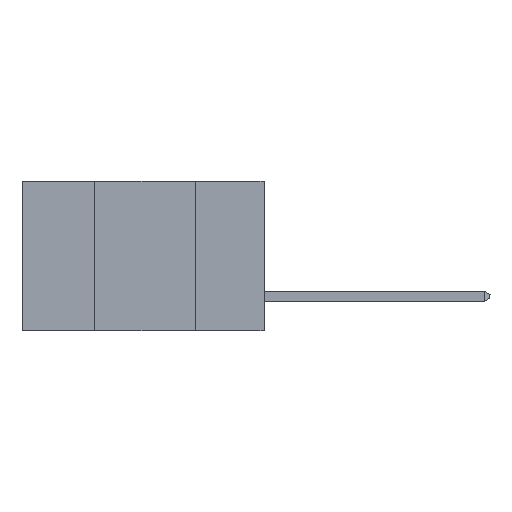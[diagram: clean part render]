
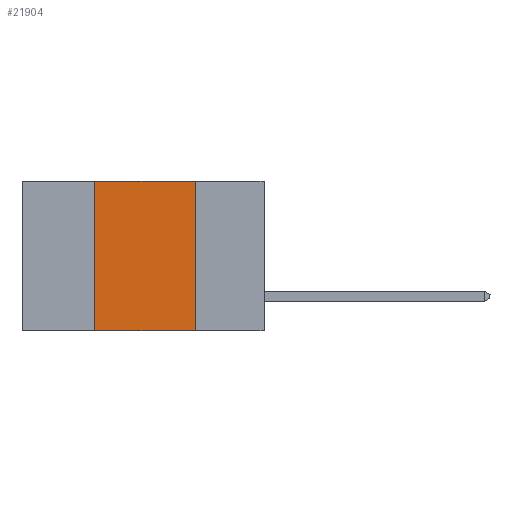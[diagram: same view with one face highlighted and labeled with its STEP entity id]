
A CAD part, left-side view. The second image highlights one B-rep face of the part: STEP entity #21904.
In plain terms, the highlighted planar face has unit normal (-1, 0, 0).
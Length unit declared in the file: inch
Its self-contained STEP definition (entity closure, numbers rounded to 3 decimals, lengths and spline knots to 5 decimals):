
#374 = VERTEX_POINT ( 'NONE', #4082 ) ;
#477 = DIRECTION ( 'NONE',  ( 0., -1., 0. ) ) ;
#605 = DIRECTION ( 'NONE',  ( 0., 0., -1. ) ) ;
#688 = EDGE_CURVE ( 'NONE', #2440, #374, #1144, .T. ) ;
#1144 = LINE ( 'NONE', #6631, #23413 ) ;
#1272 = ORIENTED_EDGE ( 'NONE', *, *, #688, .T. ) ;
#1585 = VECTOR ( 'NONE', #17593, 39.37008 ) ;
#1866 = EDGE_CURVE ( 'NONE', #2440, #13167, #24547, .T. ) ;
#2440 = VERTEX_POINT ( 'NONE', #23656 ) ;
#2526 = CARTESIAN_POINT ( 'NONE',  ( 0., 0.42, 0. ) ) ;
#2597 = LINE ( 'NONE', #20022, #15377 ) ;
#2714 = EDGE_LOOP ( 'NONE', ( #3973, #21644, #3188, #1272 ) ) ;
#3188 = ORIENTED_EDGE ( 'NONE', *, *, #1866, .F. ) ;
#3973 = ORIENTED_EDGE ( 'NONE', *, *, #20418, .F. ) ;
#4069 = VERTEX_POINT ( 'NONE', #12179 ) ;
#4082 = CARTESIAN_POINT ( 'NONE',  ( 0., 0.17, -0.37 ) ) ;
#4634 = CARTESIAN_POINT ( 'NONE',  ( 0., 0.6, 0. ) ) ;
#5079 = FACE_OUTER_BOUND ( 'NONE', #2714, .T. ) ;
#5147 = EDGE_CURVE ( 'NONE', #13167, #4069, #2597, .T. ) ;
#6631 = CARTESIAN_POINT ( 'NONE',  ( 0., 0.6, -0.37 ) ) ;
#7844 = LINE ( 'NONE', #13879, #1585 ) ;
#8522 = CARTESIAN_POINT ( 'NONE',  ( 0., 0.42, 0. ) ) ;
#8560 = AXIS2_PLACEMENT_3D ( 'NONE', #4634, #23311, #605 ) ;
#10403 = DIRECTION ( 'NONE',  ( 0., 0., 1. ) ) ;
#12096 = PLANE ( 'NONE',  #8560 ) ;
#12179 = CARTESIAN_POINT ( 'NONE',  ( 0., 0.17, 0. ) ) ;
#13167 = VERTEX_POINT ( 'NONE', #8522 ) ;
#13879 = CARTESIAN_POINT ( 'NONE',  ( 0., 0.17, 0. ) ) ;
#15377 = VECTOR ( 'NONE', #477, 39.37008 ) ;
#17403 = VECTOR ( 'NONE', #10403, 39.37008 ) ;
#17593 = DIRECTION ( 'NONE',  ( 0., 0., -1. ) ) ;
#20022 = CARTESIAN_POINT ( 'NONE',  ( 0., 0.6, 0. ) ) ;
#20418 = EDGE_CURVE ( 'NONE', #4069, #374, #7844, .T. ) ;
#21644 = ORIENTED_EDGE ( 'NONE', *, *, #5147, .F. ) ;
#21904 = ADVANCED_FACE ( 'NONE', ( #5079 ), #12096, .F. ) ;
#23311 = DIRECTION ( 'NONE',  ( 1., 0., 0. ) ) ;
#23413 = VECTOR ( 'NONE', #23890, 39.37008 ) ;
#23656 = CARTESIAN_POINT ( 'NONE',  ( 0., 0.42, -0.37 ) ) ;
#23890 = DIRECTION ( 'NONE',  ( 0., -1., 0. ) ) ;
#24547 = LINE ( 'NONE', #2526, #17403 ) ;
